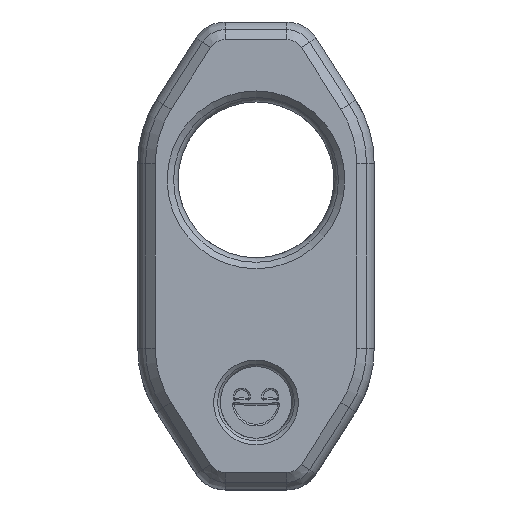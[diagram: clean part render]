
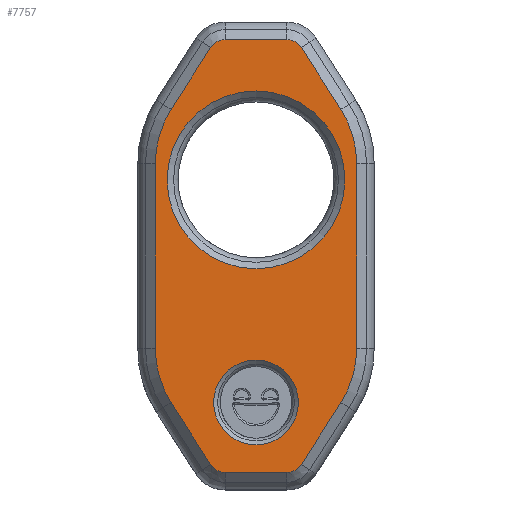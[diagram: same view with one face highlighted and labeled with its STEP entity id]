
A CAD part, front view. The second image highlights one B-rep face of the part: STEP entity #7757.
In plain terms, the highlighted planar face has unit normal (0, -1, 0).
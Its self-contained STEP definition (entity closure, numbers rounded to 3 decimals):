
#171=FACE_BOUND('',#2320,.T.);
#172=FACE_BOUND('',#2321,.T.);
#178=PLANE('',#8304);
#805=LINE('',#11414,#1297);
#806=LINE('',#11418,#1298);
#807=LINE('',#11422,#1299);
#808=LINE('',#11426,#1300);
#809=LINE('',#11430,#1301);
#810=LINE('',#11434,#1302);
#811=LINE('',#11438,#1303);
#812=LINE('',#11442,#1304);
#1297=VECTOR('',#9180,10.);
#1298=VECTOR('',#9183,10.);
#1299=VECTOR('',#9186,10.);
#1300=VECTOR('',#9189,10.);
#1301=VECTOR('',#9192,10.);
#1302=VECTOR('',#9195,10.);
#1303=VECTOR('',#9198,10.);
#1304=VECTOR('',#9201,10.);
#1814=FACE_OUTER_BOUND('',#2319,.T.);
#2319=EDGE_LOOP('',(#5286,#5287,#5288,#5289,#5290,#5291,#5292,#5293,#5294,
#5295,#5296,#5297,#5298,#5299,#5300,#5301));
#2320=EDGE_LOOP('',(#5302));
#2321=EDGE_LOOP('',(#5303));
#2824=CIRCLE('',#8272,4.84);
#2843=CIRCLE('',#8301,10.15);
#2845=CIRCLE('',#8305,2.);
#2846=CIRCLE('',#8306,11.5);
#2847=CIRCLE('',#8307,11.5);
#2848=CIRCLE('',#8308,2.);
#2849=CIRCLE('',#8309,2.);
#2850=CIRCLE('',#8310,11.5);
#2851=CIRCLE('',#8311,11.5);
#2852=CIRCLE('',#8312,2.);
#3230=VERTEX_POINT('',#11237);
#3264=VERTEX_POINT('',#11405);
#3265=VERTEX_POINT('',#11412);
#3266=VERTEX_POINT('',#11413);
#3267=VERTEX_POINT('',#11415);
#3268=VERTEX_POINT('',#11417);
#3269=VERTEX_POINT('',#11419);
#3270=VERTEX_POINT('',#11421);
#3271=VERTEX_POINT('',#11423);
#3272=VERTEX_POINT('',#11425);
#3273=VERTEX_POINT('',#11427);
#3274=VERTEX_POINT('',#11429);
#3275=VERTEX_POINT('',#11431);
#3276=VERTEX_POINT('',#11433);
#3277=VERTEX_POINT('',#11435);
#3278=VERTEX_POINT('',#11437);
#3279=VERTEX_POINT('',#11439);
#3280=VERTEX_POINT('',#11441);
#3971=EDGE_CURVE('',#3230,#3230,#2824,.T.);
#4013=EDGE_CURVE('',#3264,#3264,#2843,.T.);
#4017=EDGE_CURVE('',#3265,#3266,#805,.T.);
#4018=EDGE_CURVE('',#3265,#3267,#2845,.T.);
#4019=EDGE_CURVE('',#3267,#3268,#806,.T.);
#4020=EDGE_CURVE('',#3268,#3269,#2846,.T.);
#4021=EDGE_CURVE('',#3269,#3270,#807,.T.);
#4022=EDGE_CURVE('',#3270,#3271,#2847,.T.);
#4023=EDGE_CURVE('',#3271,#3272,#808,.T.);
#4024=EDGE_CURVE('',#3272,#3273,#2848,.T.);
#4025=EDGE_CURVE('',#3273,#3274,#809,.T.);
#4026=EDGE_CURVE('',#3275,#3274,#2849,.T.);
#4027=EDGE_CURVE('',#3276,#3275,#810,.T.);
#4028=EDGE_CURVE('',#3277,#3276,#2850,.T.);
#4029=EDGE_CURVE('',#3278,#3277,#811,.T.);
#4030=EDGE_CURVE('',#3279,#3278,#2851,.T.);
#4031=EDGE_CURVE('',#3280,#3279,#812,.T.);
#4032=EDGE_CURVE('',#3266,#3280,#2852,.T.);
#5286=ORIENTED_EDGE('',*,*,#4017,.F.);
#5287=ORIENTED_EDGE('',*,*,#4018,.T.);
#5288=ORIENTED_EDGE('',*,*,#4019,.T.);
#5289=ORIENTED_EDGE('',*,*,#4020,.T.);
#5290=ORIENTED_EDGE('',*,*,#4021,.T.);
#5291=ORIENTED_EDGE('',*,*,#4022,.T.);
#5292=ORIENTED_EDGE('',*,*,#4023,.T.);
#5293=ORIENTED_EDGE('',*,*,#4024,.T.);
#5294=ORIENTED_EDGE('',*,*,#4025,.T.);
#5295=ORIENTED_EDGE('',*,*,#4026,.F.);
#5296=ORIENTED_EDGE('',*,*,#4027,.F.);
#5297=ORIENTED_EDGE('',*,*,#4028,.F.);
#5298=ORIENTED_EDGE('',*,*,#4029,.F.);
#5299=ORIENTED_EDGE('',*,*,#4030,.F.);
#5300=ORIENTED_EDGE('',*,*,#4031,.F.);
#5301=ORIENTED_EDGE('',*,*,#4032,.F.);
#5302=ORIENTED_EDGE('',*,*,#3971,.F.);
#5303=ORIENTED_EDGE('',*,*,#4013,.F.);
#7757=ADVANCED_FACE('',(#1814,#171,#172),#178,.T.);
#8272=AXIS2_PLACEMENT_3D('',#11238,#9103,#9104);
#8301=AXIS2_PLACEMENT_3D('',#11406,#9170,#9171);
#8304=AXIS2_PLACEMENT_3D('',#11411,#9178,#9179);
#8305=AXIS2_PLACEMENT_3D('',#11416,#9181,#9182);
#8306=AXIS2_PLACEMENT_3D('',#11420,#9184,#9185);
#8307=AXIS2_PLACEMENT_3D('',#11424,#9187,#9188);
#8308=AXIS2_PLACEMENT_3D('',#11428,#9190,#9191);
#8309=AXIS2_PLACEMENT_3D('',#11432,#9193,#9194);
#8310=AXIS2_PLACEMENT_3D('',#11436,#9196,#9197);
#8311=AXIS2_PLACEMENT_3D('',#11440,#9199,#9200);
#8312=AXIS2_PLACEMENT_3D('',#11443,#9202,#9203);
#9103=DIRECTION('center_axis',(0.,-1.,0.));
#9104=DIRECTION('ref_axis',(1.,0.,0.));
#9170=DIRECTION('center_axis',(0.,-1.,0.));
#9171=DIRECTION('ref_axis',(1.,0.,0.));
#9178=DIRECTION('center_axis',(0.,-1.,0.));
#9179=DIRECTION('ref_axis',(1.,0.,0.));
#9180=DIRECTION('',(1.,0.,0.));
#9181=DIRECTION('center_axis',(0.,-1.,0.));
#9182=DIRECTION('ref_axis',(-0.481,0.,0.877));
#9183=DIRECTION('',(-0.538,0.,-0.843));
#9184=DIRECTION('center_axis',(0.,-1.,0.));
#9185=DIRECTION('ref_axis',(-0.96,0.,0.28));
#9186=DIRECTION('',(0.,0.,-1.));
#9187=DIRECTION('center_axis',(0.,-1.,0.));
#9188=DIRECTION('ref_axis',(-0.96,0.,-0.28));
#9189=DIRECTION('',(0.538,0.,-0.843));
#9190=DIRECTION('center_axis',(0.,-1.,0.));
#9191=DIRECTION('ref_axis',(-0.481,0.,-0.877));
#9192=DIRECTION('',(1.,0.,0.));
#9193=DIRECTION('center_axis',(0.,1.,0.));
#9194=DIRECTION('ref_axis',(0.481,0.,-0.877));
#9195=DIRECTION('',(-0.538,0.,-0.843));
#9196=DIRECTION('center_axis',(0.,1.,0.));
#9197=DIRECTION('ref_axis',(0.96,0.,-0.28));
#9198=DIRECTION('',(0.,0.,-1.));
#9199=DIRECTION('center_axis',(0.,1.,0.));
#9200=DIRECTION('ref_axis',(0.96,0.,0.28));
#9201=DIRECTION('',(0.538,0.,-0.843));
#9202=DIRECTION('center_axis',(0.,1.,0.));
#9203=DIRECTION('ref_axis',(0.481,0.,0.877));
#11237=CARTESIAN_POINT('',(-4.84,164.049,101.));
#11238=CARTESIAN_POINT('Origin',(0.,164.049,
101.));
#11405=CARTESIAN_POINT('',(-10.15,164.049,126.419));
#11406=CARTESIAN_POINT('Origin',(0.,164.049,
126.419));
#11411=CARTESIAN_POINT('Origin',(0.,164.049,
126.419));
#11412=CARTESIAN_POINT('',(-3.508,164.049,142.449));
#11413=CARTESIAN_POINT('',(3.508,164.049,142.449));
#11414=CARTESIAN_POINT('',(-2.258,164.049,142.449));
#11415=CARTESIAN_POINT('',(-5.195,164.049,141.524));
#11416=CARTESIAN_POINT('Origin',(-3.508,164.049,140.449));
#11417=CARTESIAN_POINT('',(-9.697,164.049,134.461));
#11418=CARTESIAN_POINT('',(-7.107,164.049,138.525));
#11419=CARTESIAN_POINT('',(-11.5,164.049,128.28));
#11420=CARTESIAN_POINT('Origin',(0.,164.049,
128.28));
#11421=CARTESIAN_POINT('',(-11.5,164.049,107.17));
#11422=CARTESIAN_POINT('',(-11.5,164.049,126.419));
#11423=CARTESIAN_POINT('',(-9.697,164.049,100.988));
#11424=CARTESIAN_POINT('Origin',(0.,164.049,
107.17));
#11425=CARTESIAN_POINT('',(-5.195,164.049,93.925));
#11426=CARTESIAN_POINT('',(-11.048,164.049,103.106));
#11427=CARTESIAN_POINT('',(-3.508,164.049,93.));
#11428=CARTESIAN_POINT('Origin',(-3.508,164.049,95.));
#11429=CARTESIAN_POINT('',(3.508,164.049,93.));
#11430=CARTESIAN_POINT('',(-6.75,164.049,93.));
#11431=CARTESIAN_POINT('',(5.195,164.049,93.925));
#11432=CARTESIAN_POINT('Origin',(3.508,164.049,95.));
#11433=CARTESIAN_POINT('',(9.697,164.049,100.988));
#11434=CARTESIAN_POINT('',(11.048,164.049,103.106));
#11435=CARTESIAN_POINT('',(11.5,164.049,107.17));
#11436=CARTESIAN_POINT('Origin',(0.,164.049,
107.17));
#11437=CARTESIAN_POINT('',(11.5,164.049,128.28));
#11438=CARTESIAN_POINT('',(11.5,164.049,126.419));
#11439=CARTESIAN_POINT('',(9.697,164.049,134.461));
#11440=CARTESIAN_POINT('Origin',(0.,164.049,
128.28));
#11441=CARTESIAN_POINT('',(5.195,164.049,141.524));
#11442=CARTESIAN_POINT('',(7.107,164.049,138.525));
#11443=CARTESIAN_POINT('Origin',(3.508,164.049,140.449));
